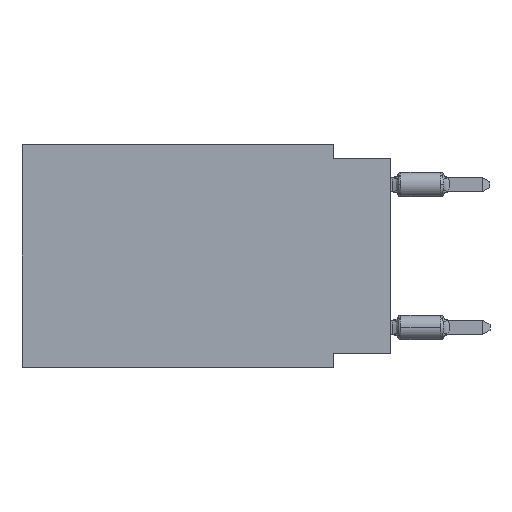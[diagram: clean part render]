
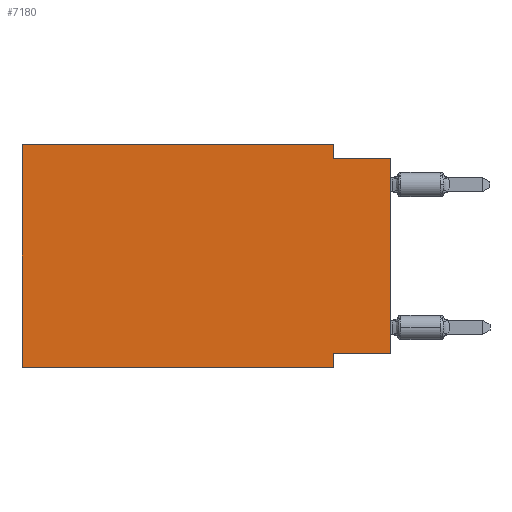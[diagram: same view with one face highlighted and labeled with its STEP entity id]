
A CAD part, left-side view. The second image highlights one B-rep face of the part: STEP entity #7180.
In plain terms, the highlighted planar face has unit normal (-1, 0, 0).
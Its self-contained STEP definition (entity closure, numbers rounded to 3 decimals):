
#113 = DIRECTION ( 'NONE',  ( 0., 0., 1. ) ) ;
#160 = LINE ( 'NONE', #7270, #1982 ) ;
#522 = AXIS2_PLACEMENT_3D ( 'NONE', #8923, #1341, #11393 ) ;
#1341 = DIRECTION ( 'NONE',  ( 1., 0., 0. ) ) ;
#1519 = CARTESIAN_POINT ( 'NONE',  ( 0., 0., 0. ) ) ;
#1715 = LINE ( 'NONE', #1519, #1926 ) ;
#1926 = VECTOR ( 'NONE', #113, 1000. ) ;
#1982 = VECTOR ( 'NONE', #13038, 1000. ) ;
#2556 = DIRECTION ( 'NONE',  ( 0., -1., 0. ) ) ;
#2992 = ORIENTED_EDGE ( 'NONE', *, *, #3568, .T. ) ;
#3130 = VERTEX_POINT ( 'NONE', #18479 ) ;
#3256 = LINE ( 'NONE', #9134, #9553 ) ;
#3260 = VERTEX_POINT ( 'NONE', #17256 ) ;
#3568 = EDGE_CURVE ( 'NONE', #8357, #3260, #14250, .T. ) ;
#4451 = ORIENTED_EDGE ( 'NONE', *, *, #5573, .F. ) ;
#4719 = VECTOR ( 'NONE', #4870, 1000. ) ;
#4870 = DIRECTION ( 'NONE',  ( 0., -1., 0. ) ) ;
#5156 = EDGE_CURVE ( 'NONE', #14954, #18743, #160, .T. ) ;
#5200 = VERTEX_POINT ( 'NONE', #12168 ) ;
#5573 = EDGE_CURVE ( 'NONE', #5200, #15546, #9041, .T. ) ;
#5971 = DIRECTION ( 'NONE',  ( 0., 0., -1. ) ) ;
#6085 = VECTOR ( 'NONE', #11160, 1000. ) ;
#6874 = EDGE_CURVE ( 'NONE', #8357, #14954, #3256, .T. ) ;
#7180 = ADVANCED_FACE ( 'NONE', ( #12999 ), #15963, .F. ) ;
#7270 = CARTESIAN_POINT ( 'NONE',  ( 0., 16.383, 0. ) ) ;
#8230 = VERTEX_POINT ( 'NONE', #14327 ) ;
#8323 = ORIENTED_EDGE ( 'NONE', *, *, #6874, .F. ) ;
#8357 = VERTEX_POINT ( 'NONE', #12490 ) ;
#8370 = CARTESIAN_POINT ( 'NONE',  ( 0., 0., -9.271 ) ) ;
#8502 = LINE ( 'NONE', #14004, #6085 ) ;
#8816 = CARTESIAN_POINT ( 'NONE',  ( 0., 16.383, 0. ) ) ;
#8923 = CARTESIAN_POINT ( 'NONE',  ( 0., 16.383, 0. ) ) ;
#9041 = LINE ( 'NONE', #13584, #4719 ) ;
#9134 = CARTESIAN_POINT ( 'NONE',  ( 0., 16.383, 0. ) ) ;
#9553 = VECTOR ( 'NONE', #10836, 1000. ) ;
#9554 = EDGE_LOOP ( 'NONE', ( #13373, #4451, #11176, #17374, #8323, #2992, #13535, #18626 ) ) ;
#10033 = CARTESIAN_POINT ( 'NONE',  ( 0., 2.54, -9.906 ) ) ;
#10321 = LINE ( 'NONE', #10033, #11922 ) ;
#10836 = DIRECTION ( 'NONE',  ( 0., 0., 1. ) ) ;
#11160 = DIRECTION ( 'NONE',  ( 0., 0., -1. ) ) ;
#11176 = ORIENTED_EDGE ( 'NONE', *, *, #11342, .F. ) ;
#11342 = EDGE_CURVE ( 'NONE', #18743, #5200, #8502, .T. ) ;
#11393 = DIRECTION ( 'NONE',  ( 0., 0., -1. ) ) ;
#11922 = VECTOR ( 'NONE', #5971, 1000. ) ;
#12168 = CARTESIAN_POINT ( 'NONE',  ( 0., 2.54, -0.635 ) ) ;
#12490 = CARTESIAN_POINT ( 'NONE',  ( 0., 16.383, -9.906 ) ) ;
#12705 = CARTESIAN_POINT ( 'NONE',  ( 0., 16.383, -9.906 ) ) ;
#12999 = FACE_OUTER_BOUND ( 'NONE', #9554, .T. ) ;
#13038 = DIRECTION ( 'NONE',  ( 0., -1., 0. ) ) ;
#13373 = ORIENTED_EDGE ( 'NONE', *, *, #16912, .T. ) ;
#13535 = ORIENTED_EDGE ( 'NONE', *, *, #14254, .F. ) ;
#13584 = CARTESIAN_POINT ( 'NONE',  ( 0., 0., -0.635 ) ) ;
#13765 = VECTOR ( 'NONE', #2556, 1000. ) ;
#14004 = CARTESIAN_POINT ( 'NONE',  ( 0., 2.54, 0. ) ) ;
#14164 = DIRECTION ( 'NONE',  ( 0., 1., 0. ) ) ;
#14250 = LINE ( 'NONE', #12705, #13765 ) ;
#14254 = EDGE_CURVE ( 'NONE', #3130, #3260, #10321, .T. ) ;
#14327 = CARTESIAN_POINT ( 'NONE',  ( 0., 0., -9.271 ) ) ;
#14461 = EDGE_CURVE ( 'NONE', #8230, #3130, #17021, .T. ) ;
#14621 = CARTESIAN_POINT ( 'NONE',  ( 0., 0., -0.635 ) ) ;
#14954 = VERTEX_POINT ( 'NONE', #8816 ) ;
#15546 = VERTEX_POINT ( 'NONE', #14621 ) ;
#15963 = PLANE ( 'NONE',  #522 ) ;
#16757 = CARTESIAN_POINT ( 'NONE',  ( 0., 2.54, 0. ) ) ;
#16912 = EDGE_CURVE ( 'NONE', #8230, #15546, #1715, .T. ) ;
#17021 = LINE ( 'NONE', #8370, #18611 ) ;
#17256 = CARTESIAN_POINT ( 'NONE',  ( 0., 2.54, -9.906 ) ) ;
#17374 = ORIENTED_EDGE ( 'NONE', *, *, #5156, .F. ) ;
#18479 = CARTESIAN_POINT ( 'NONE',  ( 0., 2.54, -9.271 ) ) ;
#18611 = VECTOR ( 'NONE', #14164, 1000. ) ;
#18626 = ORIENTED_EDGE ( 'NONE', *, *, #14461, .F. ) ;
#18743 = VERTEX_POINT ( 'NONE', #16757 ) ;
